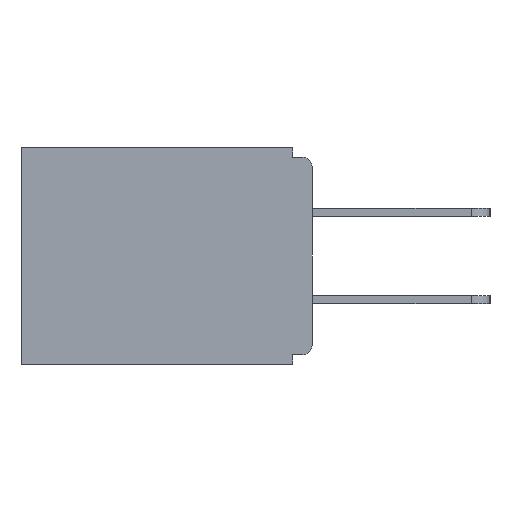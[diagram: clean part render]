
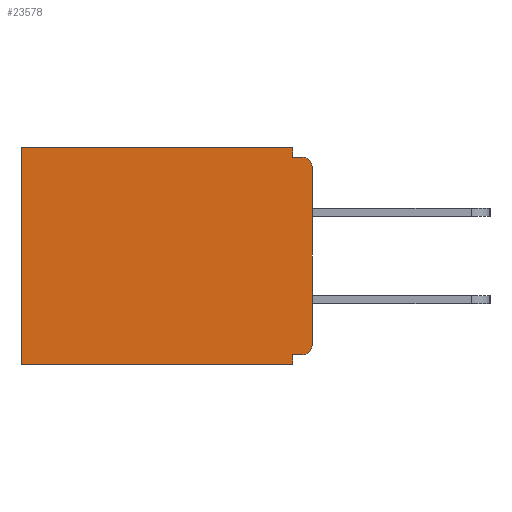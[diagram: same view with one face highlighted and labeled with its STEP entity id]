
A CAD part, left-side view. The second image highlights one B-rep face of the part: STEP entity #23578.
In plain terms, the highlighted planar face has unit normal (-1, 0, 0).
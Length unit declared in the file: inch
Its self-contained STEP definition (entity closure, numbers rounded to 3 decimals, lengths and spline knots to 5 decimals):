
#132 = EDGE_CURVE ( 'NONE', #16558, #26415, #418, .T. ) ;
#418 = LINE ( 'NONE', #20835, #23213 ) ;
#514 = PLANE ( 'NONE',  #2118 ) ;
#868 = CARTESIAN_POINT ( 'NONE',  ( 0.298, 0.031, -0.015 ) ) ;
#1236 = VECTOR ( 'NONE', #16266, 39.37008 ) ;
#1599 = VERTEX_POINT ( 'NONE', #8417 ) ;
#1794 = VECTOR ( 'NONE', #25310, 39.37008 ) ;
#2118 = AXIS2_PLACEMENT_3D ( 'NONE', #6798, #21346, #25258 ) ;
#2324 = VECTOR ( 'NONE', #11556, 39.37008 ) ;
#2606 = EDGE_CURVE ( 'NONE', #16408, #25456, #11070, .T. ) ;
#3082 = VECTOR ( 'NONE', #7934, 39.37008 ) ;
#3742 = CARTESIAN_POINT ( 'NONE',  ( 0.298, 0.031, -0.343 ) ) ;
#3754 = EDGE_CURVE ( 'NONE', #17937, #23588, #19729, .T. ) ;
#4557 = VERTEX_POINT ( 'NONE', #22205 ) ;
#5808 = CARTESIAN_POINT ( 'NONE',  ( 0.298, 0.015, -0.328 ) ) ;
#6449 = DIRECTION ( 'NONE',  ( 0., 0., -1. ) ) ;
#6775 = VECTOR ( 'NONE', #26860, 39.37008 ) ;
#6798 = CARTESIAN_POINT ( 'NONE',  ( 0.298, 0., 0. ) ) ;
#7930 = LINE ( 'NONE', #26319, #3082 ) ;
#7934 = DIRECTION ( 'NONE',  ( 0., 0., -1. ) ) ;
#8417 = CARTESIAN_POINT ( 'NONE',  ( 0.298, 0., -0.03 ) ) ;
#8985 = ORIENTED_EDGE ( 'NONE', *, *, #22786, .T. ) ;
#9021 = CARTESIAN_POINT ( 'NONE',  ( 0.298, 0.015, -0.313 ) ) ;
#9162 = VECTOR ( 'NONE', #19474, 39.37008 ) ;
#9303 = VECTOR ( 'NONE', #22445, 39.37008 ) ;
#9319 = ORIENTED_EDGE ( 'NONE', *, *, #132, .F. ) ;
#9565 = VERTEX_POINT ( 'NONE', #14449 ) ;
#10561 = CARTESIAN_POINT ( 'NONE',  ( 0.298, 0.46, -0.343 ) ) ;
#10766 = ORIENTED_EDGE ( 'NONE', *, *, #2606, .F. ) ;
#11070 = LINE ( 'NONE', #15368, #2324 ) ;
#11093 = CARTESIAN_POINT ( 'NONE',  ( 0.298, 0.031, 0. ) ) ;
#11324 = EDGE_CURVE ( 'NONE', #16408, #9565, #20433, .T. ) ;
#11556 = DIRECTION ( 'NONE',  ( 0., 1., 0. ) ) ;
#11580 = ORIENTED_EDGE ( 'NONE', *, *, #21728, .T. ) ;
#11743 = LINE ( 'NONE', #17382, #9162 ) ;
#12794 = DIRECTION ( 'NONE',  ( -1., 0., 0. ) ) ;
#12805 = CARTESIAN_POINT ( 'NONE',  ( 0.298, 0.031, -0.343 ) ) ;
#12821 = CIRCLE ( 'NONE', #20700, 0.015 ) ;
#13273 = VERTEX_POINT ( 'NONE', #14075 ) ;
#13307 = EDGE_CURVE ( 'NONE', #1599, #13273, #12821, .T. ) ;
#14075 = CARTESIAN_POINT ( 'NONE',  ( 0.298, 0.015, -0.015 ) ) ;
#14127 = ORIENTED_EDGE ( 'NONE', *, *, #14577, .F. ) ;
#14165 = CARTESIAN_POINT ( 'NONE',  ( 0.298, 0., 0. ) ) ;
#14449 = CARTESIAN_POINT ( 'NONE',  ( 0.298, 0., -0.313 ) ) ;
#14511 = CARTESIAN_POINT ( 'NONE',  ( 0.298, 0.015, -0.03 ) ) ;
#14577 = EDGE_CURVE ( 'NONE', #1599, #9565, #11743, .T. ) ;
#15368 = CARTESIAN_POINT ( 'NONE',  ( 0.298, 0., -0.328 ) ) ;
#15411 = CARTESIAN_POINT ( 'NONE',  ( 0.298, 0.031, -0.328 ) ) ;
#15852 = EDGE_CURVE ( 'NONE', #23588, #13273, #17988, .T. ) ;
#16266 = DIRECTION ( 'NONE',  ( 0., 1., 0. ) ) ;
#16408 = VERTEX_POINT ( 'NONE', #5808 ) ;
#16558 = VERTEX_POINT ( 'NONE', #12805 ) ;
#16635 = CARTESIAN_POINT ( 'NONE',  ( 0.298, 0.031, -0.343 ) ) ;
#16795 = DIRECTION ( 'NONE',  ( 0., 1., 0. ) ) ;
#16825 = CARTESIAN_POINT ( 'NONE',  ( 0.298, 0., -0.015 ) ) ;
#17382 = CARTESIAN_POINT ( 'NONE',  ( 0.298, 0., 0. ) ) ;
#17937 = VERTEX_POINT ( 'NONE', #11093 ) ;
#17988 = LINE ( 'NONE', #16825, #1794 ) ;
#18246 = ORIENTED_EDGE ( 'NONE', *, *, #13307, .T. ) ;
#19474 = DIRECTION ( 'NONE',  ( 0., 0., -1. ) ) ;
#19729 = LINE ( 'NONE', #3742, #9303 ) ;
#20433 = CIRCLE ( 'NONE', #26053, 0.015 ) ;
#20700 = AXIS2_PLACEMENT_3D ( 'NONE', #14511, #12794, #6449 ) ;
#20835 = CARTESIAN_POINT ( 'NONE',  ( 0.298, 0., -0.343 ) ) ;
#21346 = DIRECTION ( 'NONE',  ( 1., 0., 0. ) ) ;
#21591 = DIRECTION ( 'NONE',  ( 0., 0., -1. ) ) ;
#21678 = ORIENTED_EDGE ( 'NONE', *, *, #11324, .T. ) ;
#21728 = EDGE_CURVE ( 'NONE', #4557, #26415, #7930, .T. ) ;
#21868 = EDGE_CURVE ( 'NONE', #25456, #16558, #23378, .T. ) ;
#22205 = CARTESIAN_POINT ( 'NONE',  ( 0.298, 0.46, 0. ) ) ;
#22445 = DIRECTION ( 'NONE',  ( 0., 0., -1. ) ) ;
#22786 = EDGE_CURVE ( 'NONE', #17937, #4557, #23362, .T. ) ;
#23213 = VECTOR ( 'NONE', #16795, 39.37008 ) ;
#23362 = LINE ( 'NONE', #14165, #1236 ) ;
#23378 = LINE ( 'NONE', #16635, #6775 ) ;
#23578 = ADVANCED_FACE ( 'NONE', ( #23932 ), #514, .F. ) ;
#23588 = VERTEX_POINT ( 'NONE', #868 ) ;
#23758 = DIRECTION ( 'NONE',  ( -1., 0., 0. ) ) ;
#23932 = FACE_OUTER_BOUND ( 'NONE', #24727, .T. ) ;
#24018 = ORIENTED_EDGE ( 'NONE', *, *, #21868, .F. ) ;
#24283 = ORIENTED_EDGE ( 'NONE', *, *, #15852, .F. ) ;
#24727 = EDGE_LOOP ( 'NONE', ( #18246, #24283, #25889, #8985, #11580, #9319, #24018, #10766, #21678, #14127 ) ) ;
#25258 = DIRECTION ( 'NONE',  ( 0., 0., -1. ) ) ;
#25310 = DIRECTION ( 'NONE',  ( 0., -1., 0. ) ) ;
#25456 = VERTEX_POINT ( 'NONE', #15411 ) ;
#25889 = ORIENTED_EDGE ( 'NONE', *, *, #3754, .F. ) ;
#26053 = AXIS2_PLACEMENT_3D ( 'NONE', #9021, #23758, #21591 ) ;
#26319 = CARTESIAN_POINT ( 'NONE',  ( 0.298, 0.46, 0. ) ) ;
#26415 = VERTEX_POINT ( 'NONE', #10561 ) ;
#26860 = DIRECTION ( 'NONE',  ( 0., 0., -1. ) ) ;
